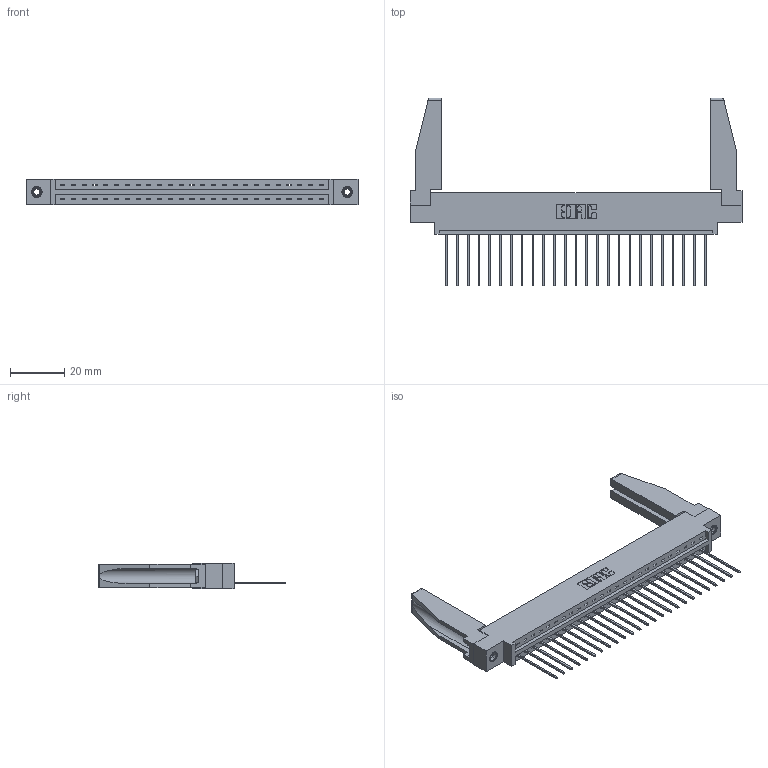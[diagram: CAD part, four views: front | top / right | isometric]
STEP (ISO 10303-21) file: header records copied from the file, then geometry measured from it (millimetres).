
FILE_DESCRIPTION (( 'STEP AP203' ), '1' );
FILE_NAME ('387-025-541-678.STEP', '2019-10-03T11:51:24', ( '' ), ( '' ), 'SwSTEP 2.0', 'SolidWorks 2016', '' );
FILE_SCHEMA (( 'CONFIG_CONTROL_DESIGN' ));
Length unit declared in the file: inch
Products named in the file (5): 307-220-078; 337 Part_0.170 Offset - 0.156 Dia-TI; 345-292-001_345-293-141; 345-250-001_345-250-001-102; 387-025-541-678
Assembly tree (30 placements, depth 2):
  387-025-541-678
    337 Part_0.170 Offset - 0.156 Dia-TI
    345-292-001_345-293-141  x25
    345-250-001_345-250-001-102  x2
    307-220-078  x2
Bounding box: 122.07 x 69.09 x 9.4 mm (x, y, z)
Volume: 16433 mm3; surface area: 17200.9 mm2
Topology: 30 solids, 30 shells, 1798 faces, 5353 edges, 3526 vertices
Faces by surface type: plane 1308, cylinder 474, cone 12, torus 4
Entity records: 23372 total; most frequent: CARTESIAN_POINT 4063, ORIENTED_EDGE 3980, DIRECTION 3464, EDGE_CURVE 1990, VECTOR 1824, LINE 1824, VERTEX_POINT 1320, AXIS2_PLACEMENT_3D 820
